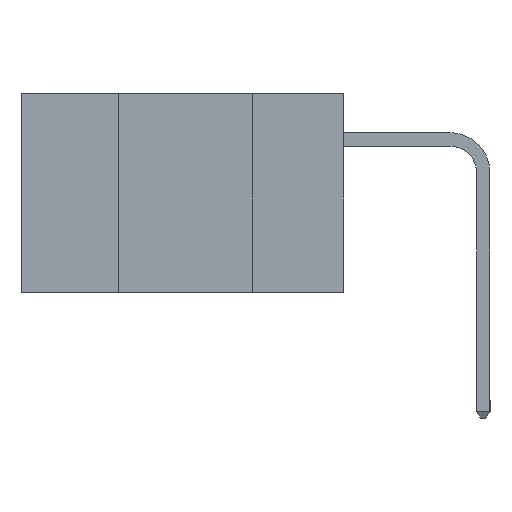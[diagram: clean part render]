
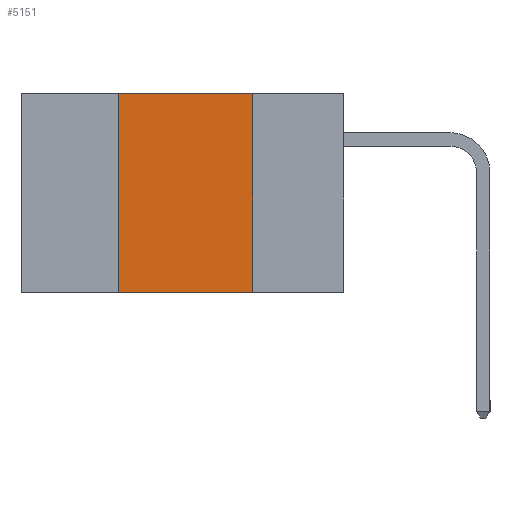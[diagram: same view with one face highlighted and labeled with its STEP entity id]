
A CAD part, left-side view. The second image highlights one B-rep face of the part: STEP entity #5151.
In plain terms, the highlighted planar face has unit normal (-1, 0, 0).
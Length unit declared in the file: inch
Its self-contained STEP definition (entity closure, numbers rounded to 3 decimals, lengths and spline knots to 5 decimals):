
#60 = EDGE_CURVE ( 'NONE', #1573, #3246, #13039, .T. ) ;
#98 = AXIS2_PLACEMENT_3D ( 'NONE', #14910, #14808, #14684 ) ;
#159 = CARTESIAN_POINT ( 'NONE',  ( 0., 0.17, -0.37 ) ) ;
#235 = CARTESIAN_POINT ( 'NONE',  ( 0., 0.42, -0.37 ) ) ;
#368 = LINE ( 'NONE', #13482, #851 ) ;
#779 = LINE ( 'NONE', #2481, #7821 ) ;
#851 = VECTOR ( 'NONE', #6280, 39.37008 ) ;
#1573 = VERTEX_POINT ( 'NONE', #2585 ) ;
#2441 = DIRECTION ( 'NONE',  ( 0., 0., -1. ) ) ;
#2481 = CARTESIAN_POINT ( 'NONE',  ( 0., 0.17, -0.37 ) ) ;
#2585 = CARTESIAN_POINT ( 'NONE',  ( 0., 0.42, -0.37 ) ) ;
#3246 = VERTEX_POINT ( 'NONE', #11825 ) ;
#3458 = ORIENTED_EDGE ( 'NONE', *, *, #60, .F. ) ;
#5151 = ADVANCED_FACE ( 'NONE', ( #9426 ), #15102, .F. ) ;
#5328 = VECTOR ( 'NONE', #18071, 39.37008 ) ;
#5883 = EDGE_CURVE ( 'NONE', #17576, #13119, #779, .T. ) ;
#6280 = DIRECTION ( 'NONE',  ( 0., -1., 0. ) ) ;
#6391 = DIRECTION ( 'NONE',  ( 0., -1., 0. ) ) ;
#7821 = VECTOR ( 'NONE', #2441, 39.37008 ) ;
#8516 = ORIENTED_EDGE ( 'NONE', *, *, #12440, .T. ) ;
#9426 = FACE_OUTER_BOUND ( 'NONE', #18790, .T. ) ;
#9774 = EDGE_CURVE ( 'NONE', #3246, #17576, #15662, .T. ) ;
#11799 = VECTOR ( 'NONE', #6391, 39.37008 ) ;
#11825 = CARTESIAN_POINT ( 'NONE',  ( 0., 0.42, 0. ) ) ;
#12134 = CARTESIAN_POINT ( 'NONE',  ( 0., 0.6, 0. ) ) ;
#12440 = EDGE_CURVE ( 'NONE', #1573, #13119, #368, .T. ) ;
#13039 = LINE ( 'NONE', #235, #5328 ) ;
#13119 = VERTEX_POINT ( 'NONE', #159 ) ;
#13482 = CARTESIAN_POINT ( 'NONE',  ( 0., 0.6, -0.37 ) ) ;
#14524 = ORIENTED_EDGE ( 'NONE', *, *, #5883, .F. ) ;
#14684 = DIRECTION ( 'NONE',  ( 0., 0., -1. ) ) ;
#14808 = DIRECTION ( 'NONE',  ( 1., 0., 0. ) ) ;
#14910 = CARTESIAN_POINT ( 'NONE',  ( 0., 0.6, 0. ) ) ;
#15102 = PLANE ( 'NONE',  #98 ) ;
#15339 = CARTESIAN_POINT ( 'NONE',  ( 0., 0.17, 0. ) ) ;
#15662 = LINE ( 'NONE', #12134, #11799 ) ;
#17576 = VERTEX_POINT ( 'NONE', #15339 ) ;
#18071 = DIRECTION ( 'NONE',  ( 0., 0., 1. ) ) ;
#18790 = EDGE_LOOP ( 'NONE', ( #14524, #18798, #3458, #8516 ) ) ;
#18798 = ORIENTED_EDGE ( 'NONE', *, *, #9774, .F. ) ;
